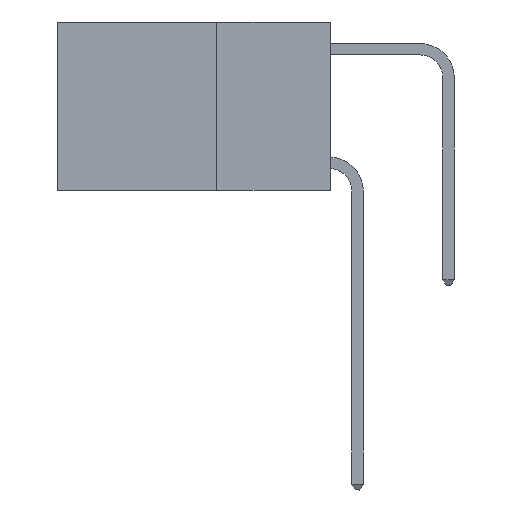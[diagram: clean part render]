
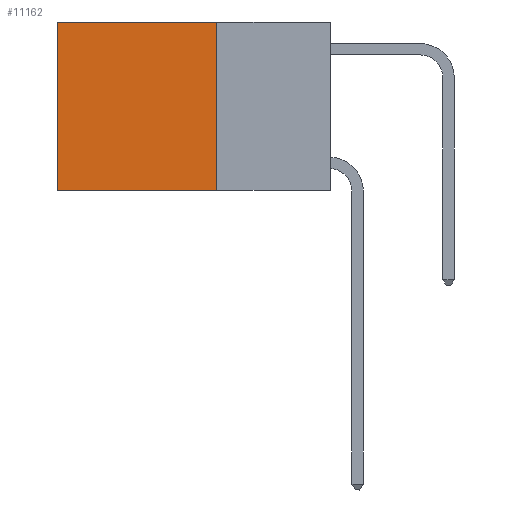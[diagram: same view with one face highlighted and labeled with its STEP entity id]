
A CAD part, left-side view. The second image highlights one B-rep face of the part: STEP entity #11162.
In plain terms, the highlighted planar face has unit normal (-1, 0, 0).
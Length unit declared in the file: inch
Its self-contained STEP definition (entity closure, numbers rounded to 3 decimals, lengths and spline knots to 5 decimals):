
#1090 = CARTESIAN_POINT ( 'NONE',  ( 0.2625, 0.25, 0. ) ) ;
#1787 = EDGE_CURVE ( 'NONE', #2917, #14399, #11152, .T. ) ;
#1817 = DIRECTION ( 'NONE',  ( 0., 0., -1. ) ) ;
#1914 = VECTOR ( 'NONE', #5310, 39.37008 ) ;
#2622 = CARTESIAN_POINT ( 'NONE',  ( 0.2625, 0.25, -0.37 ) ) ;
#2667 = DIRECTION ( 'NONE',  ( 0., 1., 0. ) ) ;
#2917 = VERTEX_POINT ( 'NONE', #2622 ) ;
#4240 = ORIENTED_EDGE ( 'NONE', *, *, #6557, .T. ) ;
#4638 = EDGE_LOOP ( 'NONE', ( #8083, #7281, #7057, #4240 ) ) ;
#5310 = DIRECTION ( 'NONE',  ( 0., 0., -1. ) ) ;
#5393 = CARTESIAN_POINT ( 'NONE',  ( 0.2625, 0.6, 0. ) ) ;
#5764 = EDGE_CURVE ( 'NONE', #10085, #2917, #7148, .T. ) ;
#6557 = EDGE_CURVE ( 'NONE', #10085, #18065, #17411, .T. ) ;
#7057 = ORIENTED_EDGE ( 'NONE', *, *, #5764, .F. ) ;
#7148 = LINE ( 'NONE', #1090, #1914 ) ;
#7263 = EDGE_CURVE ( 'NONE', #18065, #14399, #17374, .T. ) ;
#7275 = VECTOR ( 'NONE', #2667, 39.37008 ) ;
#7281 = ORIENTED_EDGE ( 'NONE', *, *, #1787, .F. ) ;
#7284 = AXIS2_PLACEMENT_3D ( 'NONE', #10282, #10534, #1817 ) ;
#8083 = ORIENTED_EDGE ( 'NONE', *, *, #7263, .T. ) ;
#9683 = CARTESIAN_POINT ( 'NONE',  ( 0.2625, 0.6, 0. ) ) ;
#10085 = VERTEX_POINT ( 'NONE', #18425 ) ;
#10282 = CARTESIAN_POINT ( 'NONE',  ( 0.2625, 0.25, 0. ) ) ;
#10534 = DIRECTION ( 'NONE',  ( 1., 0., 0. ) ) ;
#10669 = DIRECTION ( 'NONE',  ( 0., 1., 0. ) ) ;
#11152 = LINE ( 'NONE', #14587, #7275 ) ;
#11162 = ADVANCED_FACE ( 'NONE', ( #15561 ), #13222, .F. ) ;
#12344 = CARTESIAN_POINT ( 'NONE',  ( 0.2625, 0.6, -0.37 ) ) ;
#13222 = PLANE ( 'NONE',  #7284 ) ;
#13274 = VECTOR ( 'NONE', #14107, 39.37008 ) ;
#14107 = DIRECTION ( 'NONE',  ( 0., 0., -1. ) ) ;
#14399 = VERTEX_POINT ( 'NONE', #12344 ) ;
#14587 = CARTESIAN_POINT ( 'NONE',  ( 0.2625, 0.25, -0.37 ) ) ;
#15561 = FACE_OUTER_BOUND ( 'NONE', #4638, .T. ) ;
#16562 = CARTESIAN_POINT ( 'NONE',  ( 0.2625, 0.25, 0. ) ) ;
#17374 = LINE ( 'NONE', #9683, #13274 ) ;
#17411 = LINE ( 'NONE', #16562, #18538 ) ;
#18065 = VERTEX_POINT ( 'NONE', #5393 ) ;
#18425 = CARTESIAN_POINT ( 'NONE',  ( 0.2625, 0.25, 0. ) ) ;
#18538 = VECTOR ( 'NONE', #10669, 39.37008 ) ;
